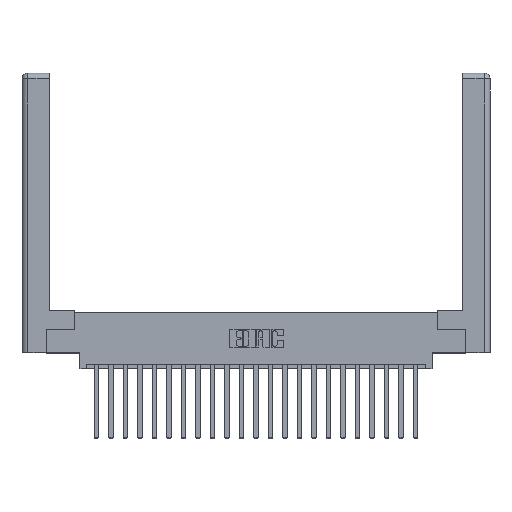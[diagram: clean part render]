
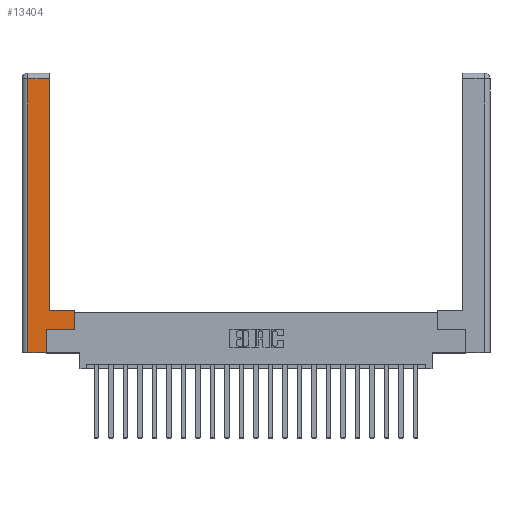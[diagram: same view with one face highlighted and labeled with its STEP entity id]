
A CAD part, top view. The second image highlights one B-rep face of the part: STEP entity #13404.
In plain terms, the highlighted planar face has unit normal (0, 0, 1).
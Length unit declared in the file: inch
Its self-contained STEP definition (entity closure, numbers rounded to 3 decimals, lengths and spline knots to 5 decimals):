
#379 = VECTOR ( 'NONE', #22875, 39.37008 ) ;
#827 = CARTESIAN_POINT ( 'NONE',  ( 0.295, 0.45, 0. ) ) ;
#905 = DIRECTION ( 'NONE',  ( 1., 0., 0. ) ) ;
#936 = EDGE_CURVE ( 'NONE', #6046, #4833, #7563, .T. ) ;
#1040 = EDGE_CURVE ( 'NONE', #5818, #14894, #2584, .T. ) ;
#2128 = DIRECTION ( 'NONE',  ( 1., 0., 0. ) ) ;
#2293 = CARTESIAN_POINT ( 'NONE',  ( 0., 0., 0. ) ) ;
#2584 = LINE ( 'NONE', #9174, #8127 ) ;
#2624 = CARTESIAN_POINT ( 'NONE',  ( 0.0615, 2.94, 0. ) ) ;
#2982 = LINE ( 'NONE', #22279, #9377 ) ;
#4787 = CARTESIAN_POINT ( 'NONE',  ( 0.565, 0.45, 0. ) ) ;
#4833 = VERTEX_POINT ( 'NONE', #4787 ) ;
#5336 = CARTESIAN_POINT ( 'NONE',  ( 0.0615, 0., 0. ) ) ;
#5818 = VERTEX_POINT ( 'NONE', #5336 ) ;
#5988 = ORIENTED_EDGE ( 'NONE', *, *, #1040, .T. ) ;
#6046 = VERTEX_POINT ( 'NONE', #14868 ) ;
#6274 = CARTESIAN_POINT ( 'NONE',  ( 0.265, 0., 0. ) ) ;
#7007 = LINE ( 'NONE', #7939, #17000 ) ;
#7141 = VERTEX_POINT ( 'NONE', #7990 ) ;
#7351 = ORIENTED_EDGE ( 'NONE', *, *, #19371, .T. ) ;
#7563 = LINE ( 'NONE', #19248, #379 ) ;
#7939 = CARTESIAN_POINT ( 'NONE',  ( 0.565, 0.245, 0. ) ) ;
#7990 = CARTESIAN_POINT ( 'NONE',  ( 0.265, 0.245, 0. ) ) ;
#8127 = VECTOR ( 'NONE', #2128, 39.37008 ) ;
#8282 = EDGE_CURVE ( 'NONE', #14894, #7141, #9118, .T. ) ;
#8449 = LINE ( 'NONE', #12693, #22572 ) ;
#8552 = VERTEX_POINT ( 'NONE', #827 ) ;
#9118 = LINE ( 'NONE', #22194, #20512 ) ;
#9174 = CARTESIAN_POINT ( 'NONE',  ( 0.265, 0., 0. ) ) ;
#9181 = PLANE ( 'NONE',  #18875 ) ;
#9377 = VECTOR ( 'NONE', #11814, 39.37008 ) ;
#9471 = VERTEX_POINT ( 'NONE', #20860 ) ;
#10446 = VECTOR ( 'NONE', #20199, 39.37008 ) ;
#10501 = VECTOR ( 'NONE', #17553, 39.37008 ) ;
#10577 = ORIENTED_EDGE ( 'NONE', *, *, #18532, .T. ) ;
#10948 = DIRECTION ( 'NONE',  ( -1., 0., 0. ) ) ;
#11814 = DIRECTION ( 'NONE',  ( 0., 1., 0. ) ) ;
#12500 = ORIENTED_EDGE ( 'NONE', *, *, #14316, .T. ) ;
#12693 = CARTESIAN_POINT ( 'NONE',  ( 0.0615, 2.94, 0. ) ) ;
#13404 = ADVANCED_FACE ( 'NONE', ( #20537 ), #9181, .F. ) ;
#13727 = EDGE_LOOP ( 'NONE', ( #20089, #7351, #21480, #5988, #20310, #12500, #18583, #10577 ) ) ;
#13922 = CARTESIAN_POINT ( 'NONE',  ( 0.0615, 0., 0. ) ) ;
#13996 = DIRECTION ( 'NONE',  ( -1., 0., 0. ) ) ;
#14316 = EDGE_CURVE ( 'NONE', #7141, #6046, #7007, .T. ) ;
#14868 = CARTESIAN_POINT ( 'NONE',  ( 0.565, 0.245, 0. ) ) ;
#14894 = VERTEX_POINT ( 'NONE', #6274 ) ;
#16563 = EDGE_CURVE ( 'NONE', #22848, #5818, #19943, .T. ) ;
#17000 = VECTOR ( 'NONE', #905, 39.37008 ) ;
#17229 = EDGE_CURVE ( 'NONE', #8552, #9471, #2982, .T. ) ;
#17382 = LINE ( 'NONE', #18157, #10446 ) ;
#17553 = DIRECTION ( 'NONE',  ( 0., -1., 0. ) ) ;
#18157 = CARTESIAN_POINT ( 'NONE',  ( 0.295, 0.45, 0. ) ) ;
#18532 = EDGE_CURVE ( 'NONE', #4833, #8552, #17382, .T. ) ;
#18583 = ORIENTED_EDGE ( 'NONE', *, *, #936, .T. ) ;
#18731 = DIRECTION ( 'NONE',  ( 0., 1., 0. ) ) ;
#18875 = AXIS2_PLACEMENT_3D ( 'NONE', #2293, #21559, #10948 ) ;
#19248 = CARTESIAN_POINT ( 'NONE',  ( 0.565, 0.45, 0. ) ) ;
#19371 = EDGE_CURVE ( 'NONE', #9471, #22848, #8449, .T. ) ;
#19943 = LINE ( 'NONE', #13922, #10501 ) ;
#20089 = ORIENTED_EDGE ( 'NONE', *, *, #17229, .T. ) ;
#20199 = DIRECTION ( 'NONE',  ( -1., 0., 0. ) ) ;
#20310 = ORIENTED_EDGE ( 'NONE', *, *, #8282, .T. ) ;
#20512 = VECTOR ( 'NONE', #18731, 39.37008 ) ;
#20537 = FACE_OUTER_BOUND ( 'NONE', #13727, .T. ) ;
#20860 = CARTESIAN_POINT ( 'NONE',  ( 0.295, 2.94, 0. ) ) ;
#21480 = ORIENTED_EDGE ( 'NONE', *, *, #16563, .T. ) ;
#21559 = DIRECTION ( 'NONE',  ( 0., 0., -1. ) ) ;
#22194 = CARTESIAN_POINT ( 'NONE',  ( 0.265, 0.245, 0. ) ) ;
#22279 = CARTESIAN_POINT ( 'NONE',  ( 0.295, 3., 0. ) ) ;
#22572 = VECTOR ( 'NONE', #13996, 39.37008 ) ;
#22848 = VERTEX_POINT ( 'NONE', #2624 ) ;
#22875 = DIRECTION ( 'NONE',  ( 0., 1., 0. ) ) ;
